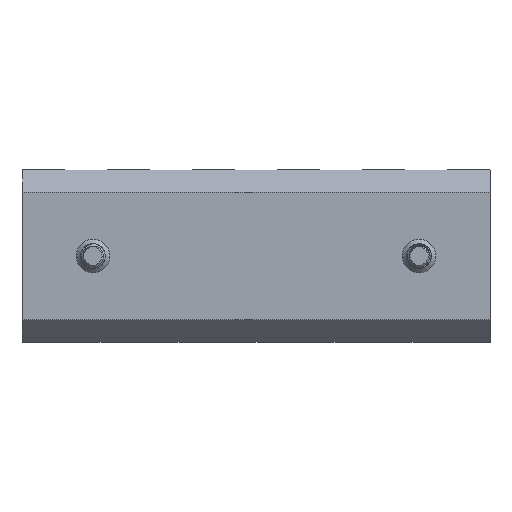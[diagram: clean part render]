
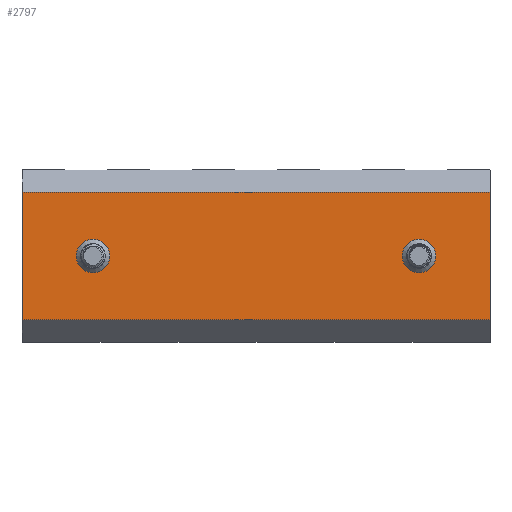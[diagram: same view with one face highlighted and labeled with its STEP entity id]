
A CAD part, left-side view. The second image highlights one B-rep face of the part: STEP entity #2797.
In plain terms, the highlighted planar face has unit normal (-1, 0, 0).
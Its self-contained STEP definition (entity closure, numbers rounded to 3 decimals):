
#35=FACE_BOUND('',#451,.T.);
#36=FACE_BOUND('',#452,.T.);
#96=PLANE('',#3019);
#288=FACE_OUTER_BOUND('',#450,.T.);
#450=EDGE_LOOP('',(#2550,#2551,#2552,#2553));
#451=EDGE_LOOP('',(#2554));
#452=EDGE_LOOP('',(#2555));
#489=CIRCLE('',#2978,2.05);
#490=CIRCLE('',#2980,2.05);
#776=LINE('',#11065,#991);
#850=LINE('',#11209,#1065);
#852=LINE('',#11213,#1067);
#853=LINE('',#11214,#1068);
#991=VECTOR('',#3482,10.);
#1065=VECTOR('',#3620,10.);
#1067=VECTOR('',#3624,10.);
#1068=VECTOR('',#3625,10.);
#1280=VERTEX_POINT('',#11033);
#1281=VERTEX_POINT('',#11037);
#1291=VERTEX_POINT('',#11062);
#1292=VERTEX_POINT('',#11064);
#1330=VERTEX_POINT('',#11208);
#1331=VERTEX_POINT('',#11212);
#1650=EDGE_CURVE('',#1280,#1280,#489,.T.);
#1652=EDGE_CURVE('',#1281,#1281,#490,.T.);
#1665=EDGE_CURVE('',#1292,#1291,#776,.T.);
#1739=EDGE_CURVE('',#1330,#1292,#850,.T.);
#1741=EDGE_CURVE('',#1331,#1291,#852,.T.);
#1742=EDGE_CURVE('',#1330,#1331,#853,.T.);
#2550=ORIENTED_EDGE('',*,*,#1665,.T.);
#2551=ORIENTED_EDGE('',*,*,#1741,.F.);
#2552=ORIENTED_EDGE('',*,*,#1742,.F.);
#2553=ORIENTED_EDGE('',*,*,#1739,.T.);
#2554=ORIENTED_EDGE('',*,*,#1650,.T.);
#2555=ORIENTED_EDGE('',*,*,#1652,.T.);
#2797=ADVANCED_FACE('',(#288,#35,#36),#96,.T.);
#2978=AXIS2_PLACEMENT_3D('',#11034,#3454,#3455);
#2980=AXIS2_PLACEMENT_3D('',#11038,#3459,#3460);
#3019=AXIS2_PLACEMENT_3D('',#11211,#3622,#3623);
#3454=DIRECTION('center_axis',(1.,0.,0.));
#3455=DIRECTION('ref_axis',(0.,1.,0.));
#3459=DIRECTION('center_axis',(1.,0.,0.));
#3460=DIRECTION('ref_axis',(0.,1.,0.));
#3482=DIRECTION('',(0.,0.,1.));
#3620=DIRECTION('',(0.,-1.,0.));
#3622=DIRECTION('center_axis',(-1.,0.,0.));
#3623=DIRECTION('ref_axis',(0.,0.,
-1.));
#3624=DIRECTION('',(0.,-1.,0.));
#3625=DIRECTION('',(0.,0.,1.));
#11033=CARTESIAN_POINT('',(0.,38.05,0.));
#11034=CARTESIAN_POINT('Origin',(0.,40.1,
0.));
#11037=CARTESIAN_POINT('',(0.,-2.05,0.));
#11038=CARTESIAN_POINT('Origin',(0.,0.,0.));
#11062=CARTESIAN_POINT('',(0.,-8.728,7.836));
#11064=CARTESIAN_POINT('',(0.,-8.728,-7.836));
#11065=CARTESIAN_POINT('',(0.,-8.728,3.918));
#11208=CARTESIAN_POINT('',(0.,48.828,-7.836));
#11209=CARTESIAN_POINT('',(0.,48.828,-7.836));
#11211=CARTESIAN_POINT('Origin',(0.,48.828,
7.836));
#11212=CARTESIAN_POINT('',(0.,48.828,7.836));
#11213=CARTESIAN_POINT('',(0.,48.828,7.836));
#11214=CARTESIAN_POINT('',(0.,48.828,-7.836));
